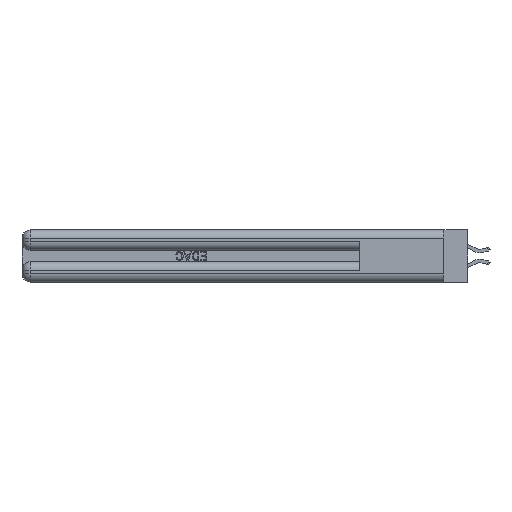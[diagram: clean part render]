
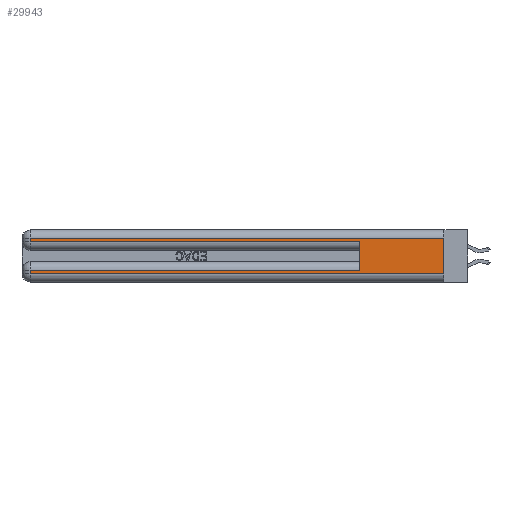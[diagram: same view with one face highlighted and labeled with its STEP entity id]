
A CAD part, left-side view. The second image highlights one B-rep face of the part: STEP entity #29943.
In plain terms, the highlighted planar face has unit normal (-1, 0, 0).
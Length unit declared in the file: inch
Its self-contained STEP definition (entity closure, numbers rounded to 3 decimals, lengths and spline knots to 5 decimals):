
#428 = DIRECTION ( 'NONE',  ( 0., -1., 0. ) ) ;
#1022 = DIRECTION ( 'NONE',  ( 0., 1., 0. ) ) ;
#3747 = VECTOR ( 'NONE', #37265, 39.37008 ) ;
#3917 = DIRECTION ( 'NONE',  ( 0., -1., 0. ) ) ;
#5181 = ORIENTED_EDGE ( 'NONE', *, *, #16302, .F. ) ;
#6301 = PLANE ( 'NONE',  #8105 ) ;
#6303 = CARTESIAN_POINT ( 'NONE',  ( 0., 2.94, 0.06 ) ) ;
#6330 = ORIENTED_EDGE ( 'NONE', *, *, #35034, .T. ) ;
#7452 = DIRECTION ( 'NONE',  ( 0., 0., -1. ) ) ;
#8105 = AXIS2_PLACEMENT_3D ( 'NONE', #27474, #30443, #12422 ) ;
#8225 = EDGE_CURVE ( 'NONE', #9137, #21220, #22359, .T. ) ;
#8561 = VECTOR ( 'NONE', #1022, 39.37008 ) ;
#8853 = EDGE_CURVE ( 'NONE', #22494, #31463, #24645, .T. ) ;
#8939 = VECTOR ( 'NONE', #3917, 39.37008 ) ;
#9137 = VERTEX_POINT ( 'NONE', #29717 ) ;
#9345 = CARTESIAN_POINT ( 'NONE',  ( 0., 2.94, 0.285 ) ) ;
#10252 = CARTESIAN_POINT ( 'NONE',  ( 0., 2.94, 0.37 ) ) ;
#10299 = EDGE_CURVE ( 'NONE', #21220, #26732, #23056, .T. ) ;
#11935 = LINE ( 'NONE', #10252, #3747 ) ;
#12401 = EDGE_CURVE ( 'NONE', #26732, #24119, #38217, .T. ) ;
#12422 = DIRECTION ( 'NONE',  ( 0., 0., -1. ) ) ;
#13783 = CARTESIAN_POINT ( 'NONE',  ( 0., 0., 0.31 ) ) ;
#14304 = VECTOR ( 'NONE', #21939, 39.37008 ) ;
#14361 = VECTOR ( 'NONE', #428, 39.37008 ) ;
#16302 = EDGE_CURVE ( 'NONE', #9137, #29172, #27808, .T. ) ;
#16993 = ORIENTED_EDGE ( 'NONE', *, *, #25737, .F. ) ;
#17512 = EDGE_LOOP ( 'NONE', ( #16993, #27140, #23231, #6330, #5181, #22195, #37166, #17796 ) ) ;
#17776 = DIRECTION ( 'NONE',  ( 0., 0., 1. ) ) ;
#17796 = ORIENTED_EDGE ( 'NONE', *, *, #12401, .T. ) ;
#18833 = CARTESIAN_POINT ( 'NONE',  ( 0., 0., 0.06 ) ) ;
#18906 = CARTESIAN_POINT ( 'NONE',  ( 0., 0., 0.085 ) ) ;
#20067 = DIRECTION ( 'NONE',  ( 0., 0., -1. ) ) ;
#21220 = VERTEX_POINT ( 'NONE', #28468 ) ;
#21299 = LINE ( 'NONE', #26095, #29216 ) ;
#21939 = DIRECTION ( 'NONE',  ( 0., 1., 0. ) ) ;
#22195 = ORIENTED_EDGE ( 'NONE', *, *, #8225, .T. ) ;
#22359 = LINE ( 'NONE', #18906, #14304 ) ;
#22425 = CARTESIAN_POINT ( 'NONE',  ( 0., 0., 0.31 ) ) ;
#22494 = VERTEX_POINT ( 'NONE', #13783 ) ;
#23056 = LINE ( 'NONE', #34666, #23988 ) ;
#23231 = ORIENTED_EDGE ( 'NONE', *, *, #35062, .T. ) ;
#23988 = VECTOR ( 'NONE', #7452, 39.37008 ) ;
#24119 = VERTEX_POINT ( 'NONE', #36598 ) ;
#24645 = LINE ( 'NONE', #22425, #8561 ) ;
#25737 = EDGE_CURVE ( 'NONE', #22494, #24119, #21299, .T. ) ;
#26095 = CARTESIAN_POINT ( 'NONE',  ( 0., 0., 0.37 ) ) ;
#26732 = VERTEX_POINT ( 'NONE', #6303 ) ;
#27140 = ORIENTED_EDGE ( 'NONE', *, *, #8853, .T. ) ;
#27474 = CARTESIAN_POINT ( 'NONE',  ( 0., 0., 0.37 ) ) ;
#27808 = LINE ( 'NONE', #29697, #34748 ) ;
#28178 = FACE_OUTER_BOUND ( 'NONE', #17512, .T. ) ;
#28199 = CARTESIAN_POINT ( 'NONE',  ( 0., 0., 0.285 ) ) ;
#28468 = CARTESIAN_POINT ( 'NONE',  ( 0., 2.94, 0.085 ) ) ;
#29172 = VERTEX_POINT ( 'NONE', #38268 ) ;
#29216 = VECTOR ( 'NONE', #20067, 39.37008 ) ;
#29697 = CARTESIAN_POINT ( 'NONE',  ( 0., 0.6, 0.145 ) ) ;
#29717 = CARTESIAN_POINT ( 'NONE',  ( 0., 0.6, 0.085 ) ) ;
#29943 = ADVANCED_FACE ( 'NONE', ( #28178 ), #6301, .F. ) ;
#30443 = DIRECTION ( 'NONE',  ( 1., 0., 0. ) ) ;
#31463 = VERTEX_POINT ( 'NONE', #35353 ) ;
#31974 = LINE ( 'NONE', #28199, #8939 ) ;
#34666 = CARTESIAN_POINT ( 'NONE',  ( 0., 2.94, 0.37 ) ) ;
#34748 = VECTOR ( 'NONE', #17776, 39.37008 ) ;
#35034 = EDGE_CURVE ( 'NONE', #36868, #29172, #31974, .T. ) ;
#35062 = EDGE_CURVE ( 'NONE', #31463, #36868, #11935, .T. ) ;
#35353 = CARTESIAN_POINT ( 'NONE',  ( 0., 2.94, 0.31 ) ) ;
#36598 = CARTESIAN_POINT ( 'NONE',  ( 0., 0., 0.06 ) ) ;
#36868 = VERTEX_POINT ( 'NONE', #9345 ) ;
#37166 = ORIENTED_EDGE ( 'NONE', *, *, #10299, .T. ) ;
#37265 = DIRECTION ( 'NONE',  ( 0., 0., -1. ) ) ;
#38217 = LINE ( 'NONE', #18833, #14361 ) ;
#38268 = CARTESIAN_POINT ( 'NONE',  ( 0., 0.6, 0.285 ) ) ;
